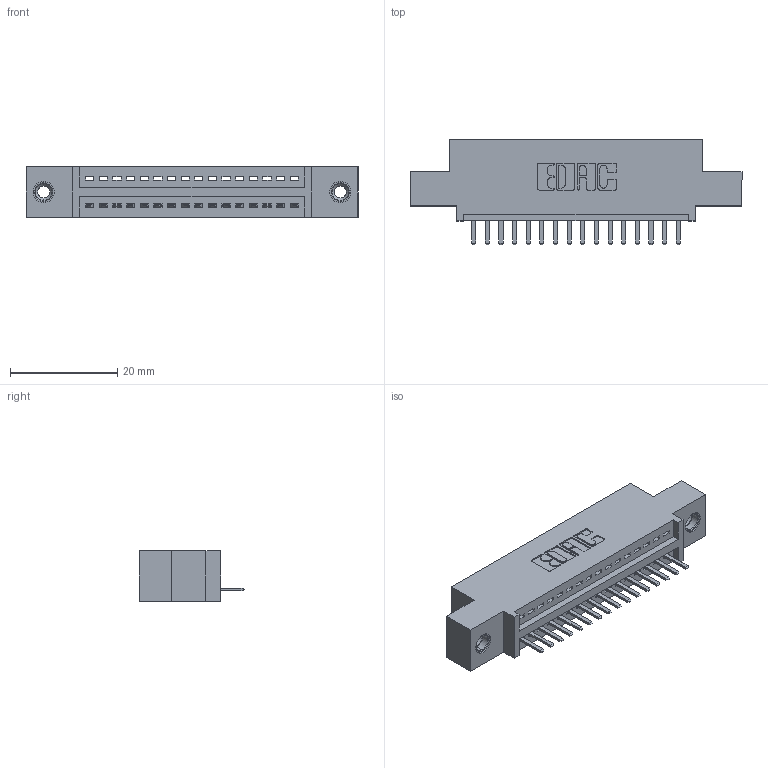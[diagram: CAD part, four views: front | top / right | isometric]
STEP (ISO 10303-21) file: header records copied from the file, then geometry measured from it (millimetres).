
FILE_DESCRIPTION (( 'STEP AP203' ), '1' );
FILE_NAME ('345-016-520-408.STEP', '2018-08-18T21:36:55', ( '' ), ( '' ), 'SwSTEP 2.0', 'SolidWorks 2016', '' );
FILE_SCHEMA (( 'CONFIG_CONTROL_DESIGN' ));
Length unit declared in the file: inch
Products named in the file (4): 345 Part_0.110 Offset - 0.156 Dia-TI; 345-292-001_345-293-120; 345-250-001_345-250-003-102; 345-016-520-408
Assembly tree (19 placements, depth 2):
  345-016-520-408
    345 Part_0.110 Offset - 0.156 Dia-TI
    345-292-001_345-293-120  x16
    345-250-001_345-250-003-102  x2
Bounding box: 61.85 x 19.68 x 9.4 mm (x, y, z)
Volume: 5535.6 mm3; surface area: 6953.4 mm2
Topology: 19 solids, 19 shells, 1182 faces, 3433 edges, 2238 vertices
Faces by surface type: plane 788, cylinder 378, cone 12, torus 4
Entity records: 16974 total; most frequent: CARTESIAN_POINT 2935, ORIENTED_EDGE 2866, DIRECTION 2615, EDGE_CURVE 1433, LINE 1213, VECTOR 1213, VERTEX_POINT 948, AXIS2_PLACEMENT_3D 701
